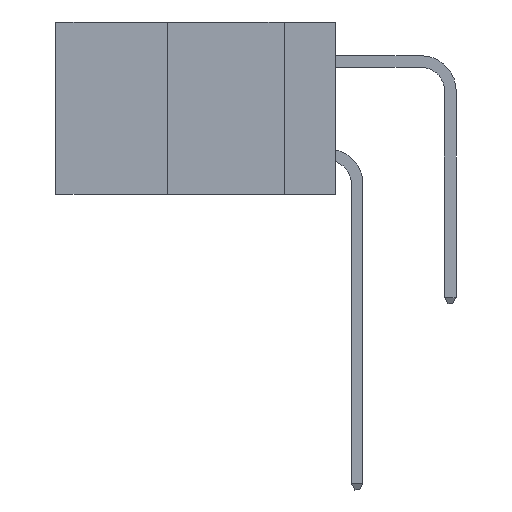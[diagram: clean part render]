
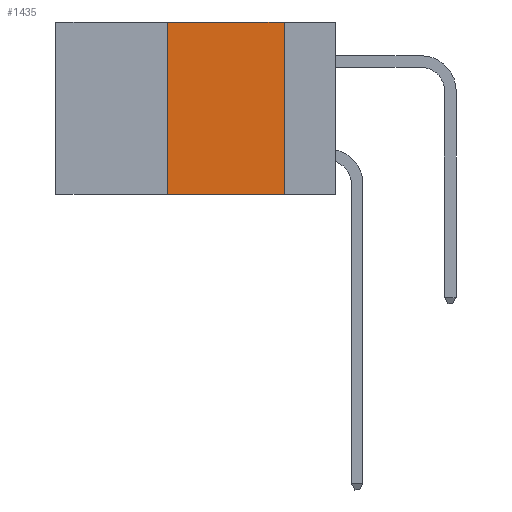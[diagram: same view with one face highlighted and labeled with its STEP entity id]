
A CAD part, left-side view. The second image highlights one B-rep face of the part: STEP entity #1435.
In plain terms, the highlighted planar face has unit normal (-1, 0, 0).
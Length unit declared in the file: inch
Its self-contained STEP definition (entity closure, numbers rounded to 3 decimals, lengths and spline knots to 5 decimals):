
#298 = FACE_OUTER_BOUND ( 'NONE', #8443, .T. ) ;
#422 = VECTOR ( 'NONE', #9913, 39.37008 ) ;
#478 = VERTEX_POINT ( 'NONE', #2101 ) ;
#810 = ORIENTED_EDGE ( 'NONE', *, *, #10152, .T. ) ;
#890 = PLANE ( 'NONE',  #6615 ) ;
#1197 = CARTESIAN_POINT ( 'NONE',  ( 0., 0.6, 0. ) ) ;
#1435 = ADVANCED_FACE ( 'NONE', ( #298 ), #890, .F. ) ;
#1531 = VECTOR ( 'NONE', #5457, 39.37008 ) ;
#2101 = CARTESIAN_POINT ( 'NONE',  ( 0., 0.11, -0.37 ) ) ;
#2454 = CARTESIAN_POINT ( 'NONE',  ( 0., 0.6, -0.37 ) ) ;
#3049 = VECTOR ( 'NONE', #10071, 39.37008 ) ;
#3513 = DIRECTION ( 'NONE',  ( 1., 0., 0. ) ) ;
#3527 = DIRECTION ( 'NONE',  ( 0., 0., -1. ) ) ;
#3718 = DIRECTION ( 'NONE',  ( 0., 0., 1. ) ) ;
#4089 = LINE ( 'NONE', #12246, #8963 ) ;
#4104 = CARTESIAN_POINT ( 'NONE',  ( 0., 0.6, 0. ) ) ;
#4764 = EDGE_CURVE ( 'NONE', #8927, #478, #5704, .T. ) ;
#5457 = DIRECTION ( 'NONE',  ( 0., -1., 0. ) ) ;
#5704 = LINE ( 'NONE', #10167, #3049 ) ;
#6615 = AXIS2_PLACEMENT_3D ( 'NONE', #1197, #3513, #3527 ) ;
#7871 = ORIENTED_EDGE ( 'NONE', *, *, #9302, .F. ) ;
#8153 = CARTESIAN_POINT ( 'NONE',  ( 0., 0.36, 0. ) ) ;
#8443 = EDGE_LOOP ( 'NONE', ( #12178, #10086, #7871, #810 ) ) ;
#8484 = VERTEX_POINT ( 'NONE', #8153 ) ;
#8927 = VERTEX_POINT ( 'NONE', #8962 ) ;
#8962 = CARTESIAN_POINT ( 'NONE',  ( 0., 0.11, 0. ) ) ;
#8963 = VECTOR ( 'NONE', #3718, 39.37008 ) ;
#9302 = EDGE_CURVE ( 'NONE', #10622, #8484, #4089, .T. ) ;
#9913 = DIRECTION ( 'NONE',  ( 0., -1., 0. ) ) ;
#10071 = DIRECTION ( 'NONE',  ( 0., 0., -1. ) ) ;
#10086 = ORIENTED_EDGE ( 'NONE', *, *, #12232, .F. ) ;
#10152 = EDGE_CURVE ( 'NONE', #10622, #478, #11795, .T. ) ;
#10167 = CARTESIAN_POINT ( 'NONE',  ( 0., 0.11, 0. ) ) ;
#10622 = VERTEX_POINT ( 'NONE', #10994 ) ;
#10913 = LINE ( 'NONE', #4104, #422 ) ;
#10994 = CARTESIAN_POINT ( 'NONE',  ( 0., 0.36, -0.37 ) ) ;
#11795 = LINE ( 'NONE', #2454, #1531 ) ;
#12178 = ORIENTED_EDGE ( 'NONE', *, *, #4764, .F. ) ;
#12232 = EDGE_CURVE ( 'NONE', #8484, #8927, #10913, .T. ) ;
#12246 = CARTESIAN_POINT ( 'NONE',  ( 0., 0.36, 0. ) ) ;
